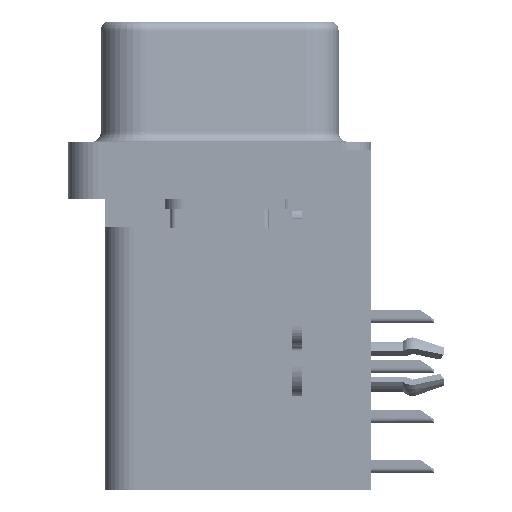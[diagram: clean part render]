
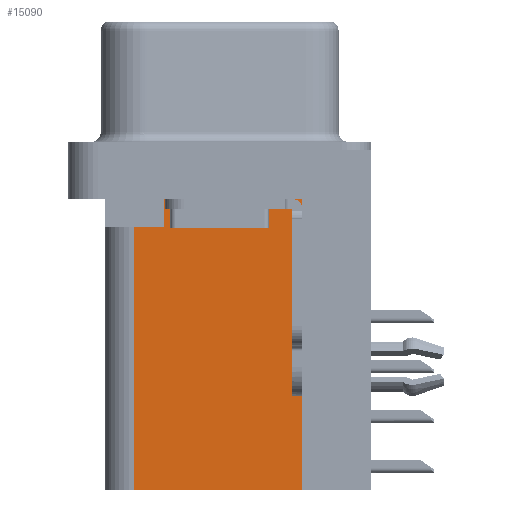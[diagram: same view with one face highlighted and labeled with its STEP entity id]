
A CAD part, left-side view. The second image highlights one B-rep face of the part: STEP entity #15090.
In plain terms, the highlighted planar face has unit normal (-1, 0, 0).
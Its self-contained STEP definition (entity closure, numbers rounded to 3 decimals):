
#1508 = VECTOR ( 'NONE', #7474, 1000. ) ;
#1615 = LINE ( 'NONE', #37371, #35965 ) ;
#1645 = CARTESIAN_POINT ( 'NONE',  ( 3.75, -4.2, -17.3 ) ) ;
#1677 = CARTESIAN_POINT ( 'NONE',  ( 3.75, 4.35, -3.9 ) ) ;
#1806 = ORIENTED_EDGE ( 'NONE', *, *, #30105, .F. ) ;
#2017 = FACE_OUTER_BOUND ( 'NONE', #5834, .T. ) ;
#3571 = DIRECTION ( 'NONE',  ( 0., 0., -1. ) ) ;
#4300 = DIRECTION ( 'NONE',  ( 0., 1., 0. ) ) ;
#4563 = EDGE_CURVE ( 'NONE', #24290, #32069, #36916, .T. ) ;
#5834 = EDGE_LOOP ( 'NONE', ( #18453, #11633, #8318, #1806, #10686, #26768 ) ) ;
#7474 = DIRECTION ( 'NONE',  ( 0., 1., 0. ) ) ;
#7862 = VECTOR ( 'NONE', #35206, 1000. ) ;
#8318 = ORIENTED_EDGE ( 'NONE', *, *, #32984, .T. ) ;
#8495 = PLANE ( 'NONE',  #39007 ) ;
#8583 = VERTEX_POINT ( 'NONE', #32519 ) ;
#10270 = DIRECTION ( 'NONE',  ( 0., 0., 1. ) ) ;
#10686 = ORIENTED_EDGE ( 'NONE', *, *, #4563, .F. ) ;
#11633 = ORIENTED_EDGE ( 'NONE', *, *, #38318, .T. ) ;
#12015 = CARTESIAN_POINT ( 'NONE',  ( 3.75, -4.2, -2.5 ) ) ;
#12752 = CARTESIAN_POINT ( 'NONE',  ( 3.75, 4.35, -17.3 ) ) ;
#12871 = VECTOR ( 'NONE', #16044, 1000. ) ;
#12994 = LINE ( 'NONE', #40032, #24508 ) ;
#13474 = EDGE_CURVE ( 'NONE', #24290, #21377, #12994, .T. ) ;
#15049 = DIRECTION ( 'NONE',  ( 0., 1., 0. ) ) ;
#15090 = ADVANCED_FACE ( 'NONE', ( #2017 ), #8495, .F. ) ;
#15651 = CARTESIAN_POINT ( 'NONE',  ( 3.75, -4.2, -17.3 ) ) ;
#15772 = EDGE_CURVE ( 'NONE', #21377, #32188, #32098, .T. ) ;
#15773 = CARTESIAN_POINT ( 'NONE',  ( 3.75, 4.35, -17.3 ) ) ;
#16044 = DIRECTION ( 'NONE',  ( 0., 0., 1. ) ) ;
#17189 = LINE ( 'NONE', #20078, #33803 ) ;
#18453 = ORIENTED_EDGE ( 'NONE', *, *, #15772, .T. ) ;
#20078 = CARTESIAN_POINT ( 'NONE',  ( 3.75, 2.85, -3.9 ) ) ;
#21377 = VERTEX_POINT ( 'NONE', #25710 ) ;
#21592 = DIRECTION ( 'NONE',  ( 1., 0., 0. ) ) ;
#21981 = VERTEX_POINT ( 'NONE', #1677 ) ;
#24290 = VERTEX_POINT ( 'NONE', #15651 ) ;
#24508 = VECTOR ( 'NONE', #10270, 1000. ) ;
#25710 = CARTESIAN_POINT ( 'NONE',  ( 3.75, -4.2, -2.5 ) ) ;
#26768 = ORIENTED_EDGE ( 'NONE', *, *, #13474, .T. ) ;
#30105 = EDGE_CURVE ( 'NONE', #32069, #21981, #39261, .T. ) ;
#31729 = CARTESIAN_POINT ( 'NONE',  ( 3.75, 2.85, -2.5 ) ) ;
#32069 = VERTEX_POINT ( 'NONE', #15773 ) ;
#32098 = LINE ( 'NONE', #12015, #7862 ) ;
#32188 = VERTEX_POINT ( 'NONE', #31729 ) ;
#32519 = CARTESIAN_POINT ( 'NONE',  ( 3.75, 2.85, -3.9 ) ) ;
#32984 = EDGE_CURVE ( 'NONE', #8583, #21981, #1615, .T. ) ;
#33803 = VECTOR ( 'NONE', #3571, 1000. ) ;
#35206 = DIRECTION ( 'NONE',  ( 0., 1., 0. ) ) ;
#35965 = VECTOR ( 'NONE', #4300, 1000. ) ;
#36916 = LINE ( 'NONE', #40385, #1508 ) ;
#37371 = CARTESIAN_POINT ( 'NONE',  ( 3.75, 0., -3.9 ) ) ;
#38318 = EDGE_CURVE ( 'NONE', #32188, #8583, #17189, .T. ) ;
#39007 = AXIS2_PLACEMENT_3D ( 'NONE', #1645, #21592, #15049 ) ;
#39261 = LINE ( 'NONE', #12752, #12871 ) ;
#40032 = CARTESIAN_POINT ( 'NONE',  ( 3.75, -4.2, -17.3 ) ) ;
#40385 = CARTESIAN_POINT ( 'NONE',  ( 3.75, -4.2, -17.3 ) ) ;
